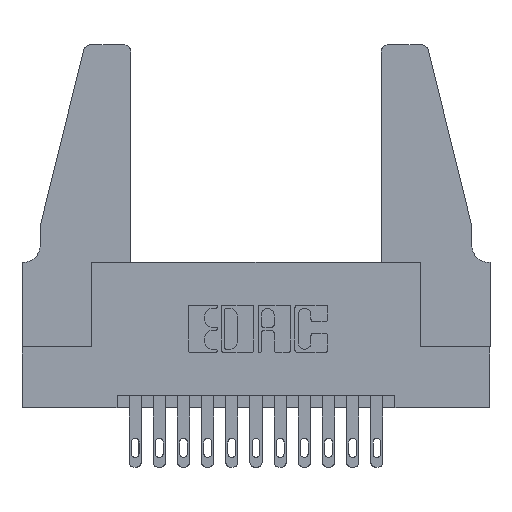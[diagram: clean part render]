
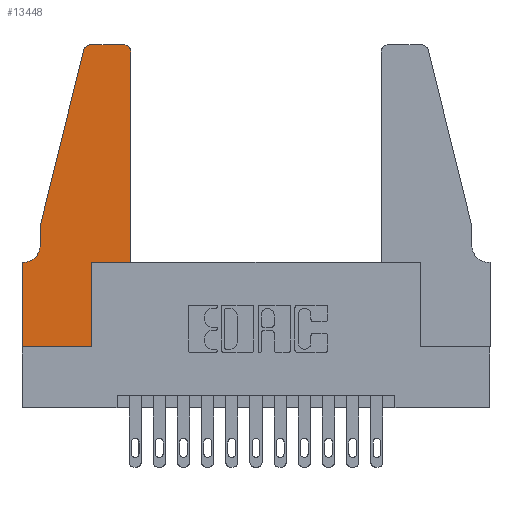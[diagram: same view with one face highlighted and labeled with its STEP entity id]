
A CAD part, top view. The second image highlights one B-rep face of the part: STEP entity #13448.
In plain terms, the highlighted planar face has unit normal (0, 0, 1).
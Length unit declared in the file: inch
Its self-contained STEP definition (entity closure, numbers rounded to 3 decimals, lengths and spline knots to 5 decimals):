
#51 = EDGE_CURVE ( 'NONE', #13824, #6531, #14782, .T. ) ;
#149 = CARTESIAN_POINT ( 'NONE',  ( 0.4505, 1.22, 0.37 ) ) ;
#211 = CARTESIAN_POINT ( 'NONE',  ( 0.0755, 0.5, 0.37 ) ) ;
#429 = VECTOR ( 'NONE', #11768, 39.37008 ) ;
#527 = CARTESIAN_POINT ( 'NONE',  ( 0.2865, 0., 0.37 ) ) ;
#588 = DIRECTION ( 'NONE',  ( 1., 0., 0. ) ) ;
#635 = VECTOR ( 'NONE', #3413, 39.37008 ) ;
#676 = CARTESIAN_POINT ( 'NONE',  ( 0.284, 1.25, 0.37 ) ) ;
#919 = VERTEX_POINT ( 'NONE', #3298 ) ;
#984 = VECTOR ( 'NONE', #14481, 39.37008 ) ;
#1083 = ORIENTED_EDGE ( 'NONE', *, *, #13258, .T. ) ;
#1151 = CARTESIAN_POINT ( 'NONE',  ( 0.4505, 0.35, 0.37 ) ) ;
#1464 = VERTEX_POINT ( 'NONE', #14290 ) ;
#1647 = LINE ( 'NONE', #7902, #14626 ) ;
#1673 = VERTEX_POINT ( 'NONE', #527 ) ;
#1819 = DIRECTION ( 'NONE',  ( 0., -1., 0. ) ) ;
#1973 = CARTESIAN_POINT ( 'NONE',  ( 0.0755, 0.5, 0.37 ) ) ;
#1993 = LINE ( 'NONE', #1151, #13472 ) ;
#2729 = ORIENTED_EDGE ( 'NONE', *, *, #4367, .T. ) ;
#2735 = AXIS2_PLACEMENT_3D ( 'NONE', #10772, #11973, #588 ) ;
#2999 = ORIENTED_EDGE ( 'NONE', *, *, #51, .T. ) ;
#3212 = LINE ( 'NONE', #11003, #6463 ) ;
#3226 = DIRECTION ( 'NONE',  ( 0., 0., 1. ) ) ;
#3231 = CARTESIAN_POINT ( 'NONE',  ( 0., 0., 0.37 ) ) ;
#3298 = CARTESIAN_POINT ( 'NONE',  ( 0., 0., 0.37 ) ) ;
#3320 = DIRECTION ( 'NONE',  ( 0., 0., -1. ) ) ;
#3413 = DIRECTION ( 'NONE',  ( -1., 0., 0. ) ) ;
#3422 = VERTEX_POINT ( 'NONE', #4869 ) ;
#3555 = LINE ( 'NONE', #4171, #984 ) ;
#3625 = EDGE_CURVE ( 'NONE', #11686, #6946, #8716, .T. ) ;
#3667 = EDGE_CURVE ( 'NONE', #12767, #1464, #13254, .T. ) ;
#3958 = DIRECTION ( 'NONE',  ( 0., 1., 0. ) ) ;
#4089 = ORIENTED_EDGE ( 'NONE', *, *, #3625, .T. ) ;
#4171 = CARTESIAN_POINT ( 'NONE',  ( 0., 0., 0.37 ) ) ;
#4367 = EDGE_CURVE ( 'NONE', #1464, #11686, #8519, .T. ) ;
#4540 = CARTESIAN_POINT ( 'NONE',  ( 0.2605, 1.25, 0.37 ) ) ;
#4741 = DIRECTION ( 'NONE',  ( 1., 0., 0. ) ) ;
#4869 = CARTESIAN_POINT ( 'NONE',  ( 0.4505, 0.35, 0.37 ) ) ;
#5355 = EDGE_CURVE ( 'NONE', #6946, #11903, #11929, .T. ) ;
#5589 = ORIENTED_EDGE ( 'NONE', *, *, #3667, .T. ) ;
#5601 = CARTESIAN_POINT ( 'NONE',  ( 0.4205, 1.22, 0.37 ) ) ;
#5658 = CARTESIAN_POINT ( 'NONE',  ( 0.284, 1.22, 0.37 ) ) ;
#5666 = DIRECTION ( 'NONE',  ( 0., 1., 0. ) ) ;
#5766 = EDGE_CURVE ( 'NONE', #6531, #8392, #1647, .T. ) ;
#5831 = CARTESIAN_POINT ( 'NONE',  ( 0.0755, 0.42, 0.37 ) ) ;
#5954 = FACE_OUTER_BOUND ( 'NONE', #10208, .T. ) ;
#6193 = CARTESIAN_POINT ( 'NONE',  ( 0., 0.35, 0.37 ) ) ;
#6301 = EDGE_CURVE ( 'NONE', #919, #1673, #3555, .T. ) ;
#6352 = ORIENTED_EDGE ( 'NONE', *, *, #6301, .T. ) ;
#6463 = VECTOR ( 'NONE', #1819, 39.37008 ) ;
#6531 = VERTEX_POINT ( 'NONE', #8828 ) ;
#6720 = ORIENTED_EDGE ( 'NONE', *, *, #12956, .T. ) ;
#6946 = VERTEX_POINT ( 'NONE', #14558 ) ;
#7027 = ORIENTED_EDGE ( 'NONE', *, *, #11275, .T. ) ;
#7902 = CARTESIAN_POINT ( 'NONE',  ( 0.0755, 0.35, 0.37 ) ) ;
#8392 = VERTEX_POINT ( 'NONE', #6193 ) ;
#8519 = LINE ( 'NONE', #4540, #635 ) ;
#8607 = LINE ( 'NONE', #10194, #11302 ) ;
#8682 = CARTESIAN_POINT ( 'NONE',  ( 0.4505, 0.35, 0.37 ) ) ;
#8716 = CIRCLE ( 'NONE', #11709, 0.03 ) ;
#8828 = CARTESIAN_POINT ( 'NONE',  ( 0.0055, 0.35, 0.37 ) ) ;
#8944 = AXIS2_PLACEMENT_3D ( 'NONE', #10172, #3320, #11137 ) ;
#9030 = EDGE_CURVE ( 'NONE', #3422, #12767, #13314, .T. ) ;
#9174 = ORIENTED_EDGE ( 'NONE', *, *, #5355, .T. ) ;
#9660 = PLANE ( 'NONE',  #2735 ) ;
#10172 = CARTESIAN_POINT ( 'NONE',  ( 0.0055, 0.42, 0.37 ) ) ;
#10194 = CARTESIAN_POINT ( 'NONE',  ( 0.2865, 0.35, 0.37 ) ) ;
#10208 = EDGE_LOOP ( 'NONE', ( #2729, #4089, #9174, #11403, #2999, #11269, #7027, #6352, #6720, #1083, #12511, #5589 ) ) ;
#10302 = DIRECTION ( 'NONE',  ( 0., -1., 0. ) ) ;
#10722 = VECTOR ( 'NONE', #10302, 39.37008 ) ;
#10772 = CARTESIAN_POINT ( 'NONE',  ( 0., 0.35, 0.37 ) ) ;
#10792 = CARTESIAN_POINT ( 'NONE',  ( 0.2865, 0.35, 0.37 ) ) ;
#11003 = CARTESIAN_POINT ( 'NONE',  ( 0.0755, 0.5, 0.37 ) ) ;
#11137 = DIRECTION ( 'NONE',  ( -1., 0., 0. ) ) ;
#11248 = DIRECTION ( 'NONE',  ( 1., 0., 0. ) ) ;
#11269 = ORIENTED_EDGE ( 'NONE', *, *, #5766, .T. ) ;
#11275 = EDGE_CURVE ( 'NONE', #8392, #919, #12532, .T. ) ;
#11302 = VECTOR ( 'NONE', #5666, 39.37008 ) ;
#11336 = VECTOR ( 'NONE', #3958, 39.37008 ) ;
#11403 = ORIENTED_EDGE ( 'NONE', *, *, #12680, .T. ) ;
#11686 = VERTEX_POINT ( 'NONE', #676 ) ;
#11709 = AXIS2_PLACEMENT_3D ( 'NONE', #5658, #3226, #11248 ) ;
#11768 = DIRECTION ( 'NONE',  ( -0.239, -0.971, 0. ) ) ;
#11903 = VERTEX_POINT ( 'NONE', #1973 ) ;
#11929 = LINE ( 'NONE', #211, #429 ) ;
#11973 = DIRECTION ( 'NONE',  ( 0., 0., 1. ) ) ;
#12511 = ORIENTED_EDGE ( 'NONE', *, *, #9030, .T. ) ;
#12532 = LINE ( 'NONE', #3231, #10722 ) ;
#12680 = EDGE_CURVE ( 'NONE', #11903, #13824, #3212, .T. ) ;
#12767 = VERTEX_POINT ( 'NONE', #149 ) ;
#12956 = EDGE_CURVE ( 'NONE', #1673, #14596, #8607, .T. ) ;
#13068 = AXIS2_PLACEMENT_3D ( 'NONE', #5601, #13617, #13525 ) ;
#13254 = CIRCLE ( 'NONE', #13068, 0.03 ) ;
#13258 = EDGE_CURVE ( 'NONE', #14596, #3422, #1993, .T. ) ;
#13314 = LINE ( 'NONE', #8682, #11336 ) ;
#13448 = ADVANCED_FACE ( 'NONE', ( #5954 ), #9660, .T. ) ;
#13472 = VECTOR ( 'NONE', #4741, 39.37008 ) ;
#13525 = DIRECTION ( 'NONE',  ( 1., 0., 0. ) ) ;
#13617 = DIRECTION ( 'NONE',  ( 0., 0., 1. ) ) ;
#13708 = DIRECTION ( 'NONE',  ( -1., 0., 0. ) ) ;
#13824 = VERTEX_POINT ( 'NONE', #5831 ) ;
#14290 = CARTESIAN_POINT ( 'NONE',  ( 0.4205, 1.25, 0.37 ) ) ;
#14481 = DIRECTION ( 'NONE',  ( 1., 0., 0. ) ) ;
#14558 = CARTESIAN_POINT ( 'NONE',  ( 0.25487, 1.22718, 0.37 ) ) ;
#14596 = VERTEX_POINT ( 'NONE', #10792 ) ;
#14626 = VECTOR ( 'NONE', #13708, 39.37008 ) ;
#14782 = CIRCLE ( 'NONE', #8944, 0.07 ) ;
